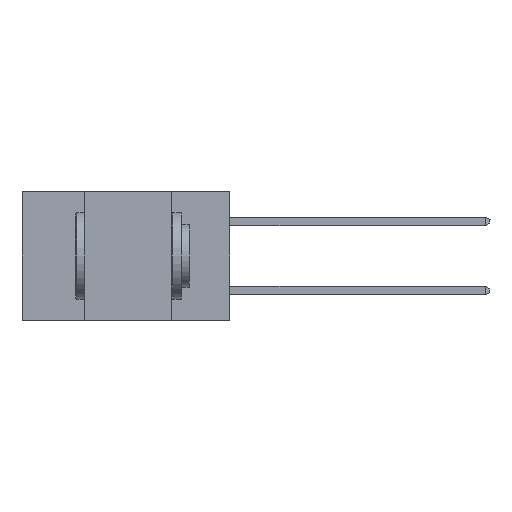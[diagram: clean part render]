
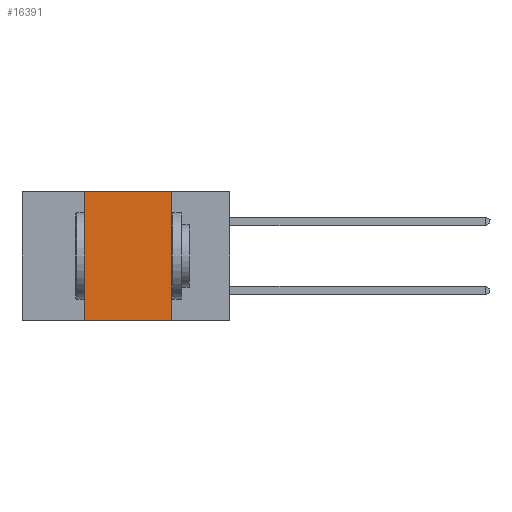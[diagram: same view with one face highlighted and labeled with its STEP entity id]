
A CAD part, left-side view. The second image highlights one B-rep face of the part: STEP entity #16391.
In plain terms, the highlighted planar face has unit normal (-1, 0, 0).
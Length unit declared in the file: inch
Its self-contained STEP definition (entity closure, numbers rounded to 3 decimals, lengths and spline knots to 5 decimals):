
#844 = CARTESIAN_POINT ( 'NONE',  ( 0., 0.42, 0. ) ) ;
#1193 = CARTESIAN_POINT ( 'NONE',  ( 0., 0.42, -0.37 ) ) ;
#1253 = FACE_OUTER_BOUND ( 'NONE', #18670, .T. ) ;
#1792 = ORIENTED_EDGE ( 'NONE', *, *, #1938, .F. ) ;
#1824 = CARTESIAN_POINT ( 'NONE',  ( 0., 0.42, -0.37 ) ) ;
#1910 = VERTEX_POINT ( 'NONE', #9833 ) ;
#1938 = EDGE_CURVE ( 'NONE', #2660, #13581, #23911, .T. ) ;
#2660 = VERTEX_POINT ( 'NONE', #1193 ) ;
#3131 = LINE ( 'NONE', #27232, #12371 ) ;
#3162 = LINE ( 'NONE', #5020, #8472 ) ;
#3197 = EDGE_CURVE ( 'NONE', #1910, #22177, #26986, .T. ) ;
#5020 = CARTESIAN_POINT ( 'NONE',  ( 0., 0.6, 0. ) ) ;
#5135 = EDGE_CURVE ( 'NONE', #13581, #1910, #3162, .T. ) ;
#5582 = VECTOR ( 'NONE', #9728, 39.37008 ) ;
#6815 = EDGE_CURVE ( 'NONE', #2660, #22177, #3131, .T. ) ;
#8472 = VECTOR ( 'NONE', #9589, 39.37008 ) ;
#8587 = ORIENTED_EDGE ( 'NONE', *, *, #6815, .T. ) ;
#9589 = DIRECTION ( 'NONE',  ( 0., -1., 0. ) ) ;
#9728 = DIRECTION ( 'NONE',  ( 0., 0., -1. ) ) ;
#9833 = CARTESIAN_POINT ( 'NONE',  ( 0., 0.17, 0. ) ) ;
#9943 = DIRECTION ( 'NONE',  ( 0., 0., -1. ) ) ;
#12371 = VECTOR ( 'NONE', #14108, 39.37008 ) ;
#13581 = VERTEX_POINT ( 'NONE', #844 ) ;
#14108 = DIRECTION ( 'NONE',  ( 0., -1., 0. ) ) ;
#15062 = VECTOR ( 'NONE', #24046, 39.37008 ) ;
#16391 = ADVANCED_FACE ( 'NONE', ( #1253 ), #24774, .F. ) ;
#17417 = CARTESIAN_POINT ( 'NONE',  ( 0., 0.17, -0.37 ) ) ;
#18670 = EDGE_LOOP ( 'NONE', ( #28054, #26826, #1792, #8587 ) ) ;
#21055 = CARTESIAN_POINT ( 'NONE',  ( 0., 0.6, 0. ) ) ;
#22177 = VERTEX_POINT ( 'NONE', #17417 ) ;
#23911 = LINE ( 'NONE', #1824, #15062 ) ;
#24046 = DIRECTION ( 'NONE',  ( 0., 0., 1. ) ) ;
#24534 = CARTESIAN_POINT ( 'NONE',  ( 0., 0.17, -0.37 ) ) ;
#24774 = PLANE ( 'NONE',  #26334 ) ;
#26334 = AXIS2_PLACEMENT_3D ( 'NONE', #21055, #27070, #9943 ) ;
#26826 = ORIENTED_EDGE ( 'NONE', *, *, #5135, .F. ) ;
#26986 = LINE ( 'NONE', #24534, #5582 ) ;
#27070 = DIRECTION ( 'NONE',  ( 1., 0., 0. ) ) ;
#27232 = CARTESIAN_POINT ( 'NONE',  ( 0., 0.6, -0.37 ) ) ;
#28054 = ORIENTED_EDGE ( 'NONE', *, *, #3197, .F. ) ;
